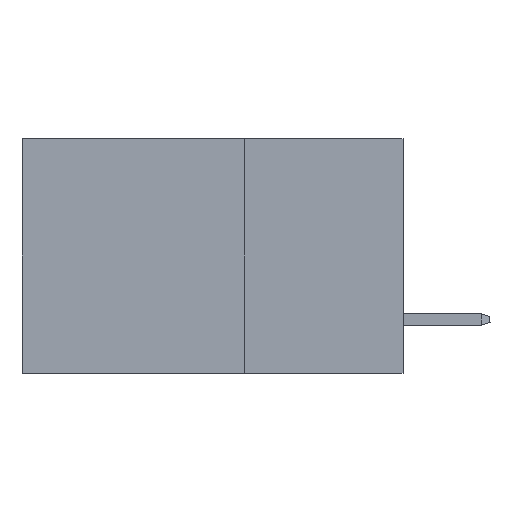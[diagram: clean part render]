
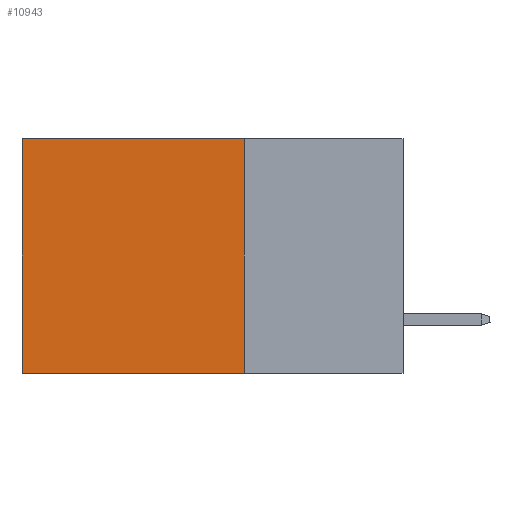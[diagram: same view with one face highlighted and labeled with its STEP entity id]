
A CAD part, left-side view. The second image highlights one B-rep face of the part: STEP entity #10943.
In plain terms, the highlighted planar face has unit normal (-1, 0, 0).
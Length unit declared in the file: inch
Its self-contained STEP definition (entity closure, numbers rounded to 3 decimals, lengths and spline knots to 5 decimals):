
#184 = EDGE_CURVE ( 'NONE', #5673, #25117, #18752, .T. ) ;
#580 = VECTOR ( 'NONE', #5931, 39.37008 ) ;
#3562 = CARTESIAN_POINT ( 'NONE',  ( 0.2875, 0.25, 0. ) ) ;
#4757 = DIRECTION ( 'NONE',  ( 1., 0., 0. ) ) ;
#5673 = VERTEX_POINT ( 'NONE', #31478 ) ;
#5931 = DIRECTION ( 'NONE',  ( 0., 1., 0. ) ) ;
#6917 = PLANE ( 'NONE',  #22583 ) ;
#7310 = CARTESIAN_POINT ( 'NONE',  ( 0.2875, 0.6, 0. ) ) ;
#7541 = CARTESIAN_POINT ( 'NONE',  ( 0.2875, 0.25, -0.37 ) ) ;
#8180 = EDGE_CURVE ( 'NONE', #8775, #8797, #25850, .T. ) ;
#8509 = EDGE_CURVE ( 'NONE', #25117, #8797, #19977, .T. ) ;
#8604 = ORIENTED_EDGE ( 'NONE', *, *, #16402, .F. ) ;
#8775 = VERTEX_POINT ( 'NONE', #29581 ) ;
#8797 = VERTEX_POINT ( 'NONE', #22101 ) ;
#9406 = DIRECTION ( 'NONE',  ( 0., 0., -1. ) ) ;
#10529 = DIRECTION ( 'NONE',  ( 0., 1., 0. ) ) ;
#10943 = ADVANCED_FACE ( 'NONE', ( #11738 ), #6917, .F. ) ;
#11738 = FACE_OUTER_BOUND ( 'NONE', #26407, .T. ) ;
#15530 = VECTOR ( 'NONE', #10529, 39.37008 ) ;
#16402 = EDGE_CURVE ( 'NONE', #5673, #8775, #18391, .T. ) ;
#18381 = VECTOR ( 'NONE', #29000, 39.37008 ) ;
#18391 = LINE ( 'NONE', #3562, #18381 ) ;
#18432 = CARTESIAN_POINT ( 'NONE',  ( 0.2875, 0.25, 0. ) ) ;
#18752 = LINE ( 'NONE', #18432, #580 ) ;
#19977 = LINE ( 'NONE', #7310, #30951 ) ;
#22101 = CARTESIAN_POINT ( 'NONE',  ( 0.2875, 0.6, -0.37 ) ) ;
#22583 = AXIS2_PLACEMENT_3D ( 'NONE', #27217, #4757, #9406 ) ;
#22963 = DIRECTION ( 'NONE',  ( 0., 0., -1. ) ) ;
#25117 = VERTEX_POINT ( 'NONE', #27489 ) ;
#25850 = LINE ( 'NONE', #7541, #15530 ) ;
#26359 = ORIENTED_EDGE ( 'NONE', *, *, #8509, .T. ) ;
#26407 = EDGE_LOOP ( 'NONE', ( #26359, #29309, #8604, #26414 ) ) ;
#26414 = ORIENTED_EDGE ( 'NONE', *, *, #184, .T. ) ;
#27217 = CARTESIAN_POINT ( 'NONE',  ( 0.2875, 0.25, 0. ) ) ;
#27489 = CARTESIAN_POINT ( 'NONE',  ( 0.2875, 0.6, 0. ) ) ;
#29000 = DIRECTION ( 'NONE',  ( 0., 0., -1. ) ) ;
#29309 = ORIENTED_EDGE ( 'NONE', *, *, #8180, .F. ) ;
#29581 = CARTESIAN_POINT ( 'NONE',  ( 0.2875, 0.25, -0.37 ) ) ;
#30951 = VECTOR ( 'NONE', #22963, 39.37008 ) ;
#31478 = CARTESIAN_POINT ( 'NONE',  ( 0.2875, 0.25, 0. ) ) ;
